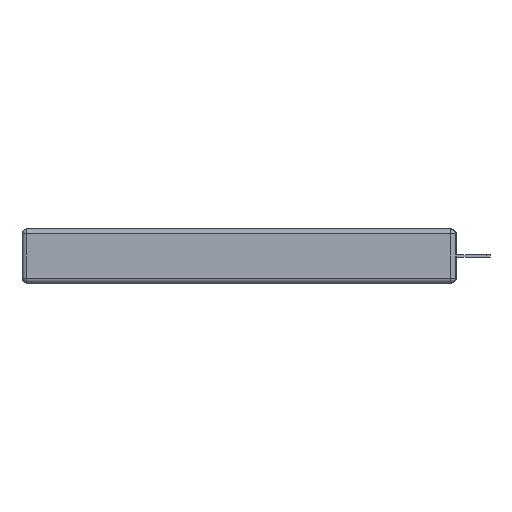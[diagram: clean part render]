
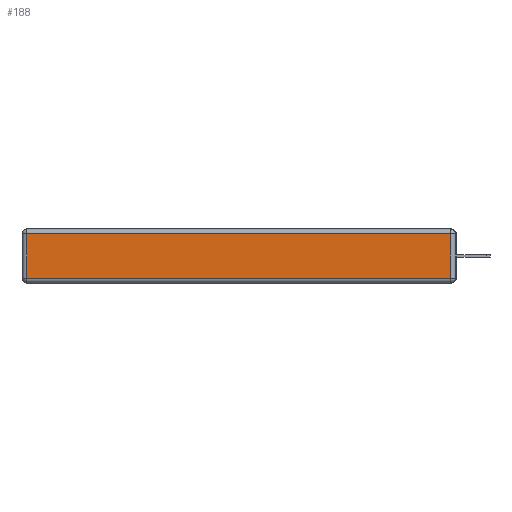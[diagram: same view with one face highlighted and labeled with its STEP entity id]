
A CAD part, left-side view. The second image highlights one B-rep face of the part: STEP entity #188.
In plain terms, the highlighted planar face has unit normal (-1, 0, 0).
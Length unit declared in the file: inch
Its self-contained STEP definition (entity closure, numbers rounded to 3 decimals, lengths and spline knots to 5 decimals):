
#188 = ADVANCED_FACE ( 'NONE', ( #6247 ), #11298, .T. ) ;
#300 = DIRECTION ( 'NONE',  ( 0., 0., 1. ) ) ;
#1705 = ORIENTED_EDGE ( 'NONE', *, *, #12350, .T. ) ;
#2024 = VERTEX_POINT ( 'NONE', #17136 ) ;
#6117 = LINE ( 'NONE', #8738, #22286 ) ;
#6247 = FACE_OUTER_BOUND ( 'NONE', #13459, .T. ) ;
#7215 = EDGE_CURVE ( 'NONE', #13857, #17717, #22027, .T. ) ;
#8738 = CARTESIAN_POINT ( 'NONE',  ( 0., 0., -0.313 ) ) ;
#9022 = LINE ( 'NONE', #20720, #25112 ) ;
#10953 = CARTESIAN_POINT ( 'NONE',  ( 0., 2.75, -0.03 ) ) ;
#11004 = CARTESIAN_POINT ( 'NONE',  ( 0., 0.03, -0.343 ) ) ;
#11298 = PLANE ( 'NONE',  #14513 ) ;
#11411 = CARTESIAN_POINT ( 'NONE',  ( 0., 0.03, -0.313 ) ) ;
#12350 = EDGE_CURVE ( 'NONE', #21602, #13857, #23342, .T. ) ;
#13110 = DIRECTION ( 'NONE',  ( 0., 0., 1. ) ) ;
#13459 = EDGE_LOOP ( 'NONE', ( #13662, #1705, #19939, #19288 ) ) ;
#13662 = ORIENTED_EDGE ( 'NONE', *, *, #18863, .T. ) ;
#13857 = VERTEX_POINT ( 'NONE', #23182 ) ;
#14513 = AXIS2_PLACEMENT_3D ( 'NONE', #25416, #23177, #300 ) ;
#17080 = DIRECTION ( 'NONE',  ( 0., -1., 0. ) ) ;
#17094 = VECTOR ( 'NONE', #19199, 39.37008 ) ;
#17136 = CARTESIAN_POINT ( 'NONE',  ( 0., 2.72, -0.313 ) ) ;
#17717 = VERTEX_POINT ( 'NONE', #23849 ) ;
#17758 = VECTOR ( 'NONE', #13110, 39.37008 ) ;
#18863 = EDGE_CURVE ( 'NONE', #2024, #21602, #6117, .T. ) ;
#19199 = DIRECTION ( 'NONE',  ( 0., 1., 0. ) ) ;
#19288 = ORIENTED_EDGE ( 'NONE', *, *, #20664, .T. ) ;
#19939 = ORIENTED_EDGE ( 'NONE', *, *, #7215, .T. ) ;
#20664 = EDGE_CURVE ( 'NONE', #17717, #2024, #9022, .T. ) ;
#20720 = CARTESIAN_POINT ( 'NONE',  ( 0., 2.72, -0.343 ) ) ;
#21602 = VERTEX_POINT ( 'NONE', #11411 ) ;
#22027 = LINE ( 'NONE', #10953, #17094 ) ;
#22286 = VECTOR ( 'NONE', #17080, 39.37008 ) ;
#23177 = DIRECTION ( 'NONE',  ( -1., 0., 0. ) ) ;
#23182 = CARTESIAN_POINT ( 'NONE',  ( 0., 0.03, -0.03 ) ) ;
#23342 = LINE ( 'NONE', #11004, #17758 ) ;
#23849 = CARTESIAN_POINT ( 'NONE',  ( 0., 2.72, -0.03 ) ) ;
#25112 = VECTOR ( 'NONE', #27071, 39.37008 ) ;
#25416 = CARTESIAN_POINT ( 'NONE',  ( 0., 0., -0.343 ) ) ;
#27071 = DIRECTION ( 'NONE',  ( 0., 0., -1. ) ) ;
